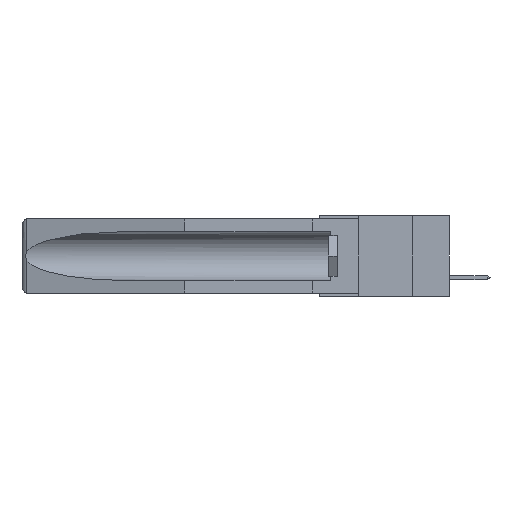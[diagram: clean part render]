
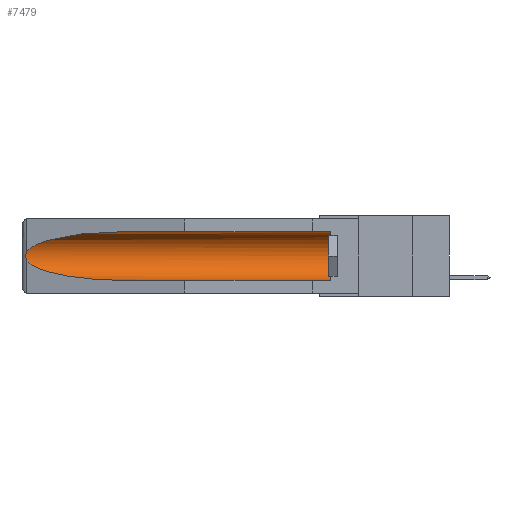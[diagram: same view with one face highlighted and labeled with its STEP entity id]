
A CAD part, left-side view. The second image highlights one B-rep face of the part: STEP entity #7479.
In plain terms, the highlighted cylindrical face has radius 2.857 mm (diameter 5.715 mm), a partial arc.
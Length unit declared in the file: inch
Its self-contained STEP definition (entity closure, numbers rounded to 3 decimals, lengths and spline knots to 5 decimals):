
#168 = CARTESIAN_POINT ( 'NONE',  ( 0.26597, 1.52961, -0.15275 ) ) ;
#580 = LINE ( 'NONE', #3867, #10991 ) ;
#1184 = VERTEX_POINT ( 'NONE', #15081 ) ;
#1246 = FACE_OUTER_BOUND ( 'NONE', #3097, .T. ) ;
#1307 = CARTESIAN_POINT ( 'NONE',  ( 0.26537, 1.52718, -0.19328 ) ) ;
#3097 = EDGE_LOOP ( 'NONE', ( #18067, #24469, #7619, #7277, #23403, #26699 ) ) ;
#3204 = CARTESIAN_POINT ( 'NONE',  ( 0.25451, 1.48313, -0.09465 ) ) ;
#3775 = DIRECTION ( 'NONE',  ( 0., 1., 0. ) ) ;
#3867 = CARTESIAN_POINT ( 'NONE',  ( 0.155, -0.30754, -0.284 ) ) ;
#3916 = CARTESIAN_POINT ( 'NONE',  ( 0.155, 0.126, -0.059 ) ) ;
#4018 = AXIS2_PLACEMENT_3D ( 'NONE', #15516, #21677, #5068 ) ;
#4229 = CARTESIAN_POINT ( 'NONE',  ( 0.155, 0.126, -0.1715 ) ) ;
#4528 = LINE ( 'NONE', #22817, #7834 ) ;
#4541 = CARTESIAN_POINT ( 'NONE',  ( 0.26537, 1.52718, -0.14972 ) ) ;
#4928 = CARTESIAN_POINT ( 'NONE',  ( 0.26537, 1.52718, -0.14972 ) ) ;
#5046 = EDGE_CURVE ( 'NONE', #12075, #1184, #12739, .T. ) ;
#5068 = DIRECTION ( 'NONE',  ( 0., 0., 1. ) ) ;
#5694 = CARTESIAN_POINT ( 'NONE',  ( 0.21114, 1.30732, -0.284 ) ) ;
#5814 = VERTEX_POINT ( 'NONE', #3916 ) ;
#6275 = EDGE_CURVE ( 'NONE', #5814, #20178, #4528, .T. ) ;
#6445 = CARTESIAN_POINT ( 'NONE',  ( 0.2675, 1.53308, -0.16763 ) ) ;
#6728 = CARTESIAN_POINT ( 'NONE',  ( 0.155, 0.126, -0.284 ) ) ;
#6777 = CYLINDRICAL_SURFACE ( 'NONE', #4018, 0.1125 ) ;
#7117 = EDGE_CURVE ( 'NONE', #11679, #12075, #21382, .T. ) ;
#7277 = ORIENTED_EDGE ( 'NONE', *, *, #25145, .F. ) ;
#7479 = ADVANCED_FACE ( 'NONE', ( #1246 ), #6777, .F. ) ;
#7619 = ORIENTED_EDGE ( 'NONE', *, *, #5046, .T. ) ;
#7834 = VECTOR ( 'NONE', #12122, 39.37008 ) ;
#8547 = CARTESIAN_POINT ( 'NONE',  ( 0.26655, 1.53094, -0.18657 ) ) ;
#8723 = CARTESIAN_POINT ( 'NONE',  ( 0.2673, 1.53269, -0.17917 ) ) ;
#9091 = CIRCLE ( 'NONE', #23106, 0.1125 ) ;
#9810 = CARTESIAN_POINT ( 'NONE',  ( 0.26537, 1.52718, -0.19328 ) ) ;
#9898 = CARTESIAN_POINT ( 'NONE',  ( 0.25451, 1.48313, -0.24835 ) ) ;
#10991 = VECTOR ( 'NONE', #3775, 39.37008 ) ;
#11486 = CARTESIAN_POINT ( 'NONE',  ( 0.155, 1.07973, -0.059 ) ) ;
#11679 = VERTEX_POINT ( 'NONE', #19149 ) ;
#12075 = VERTEX_POINT ( 'NONE', #1307 ) ;
#12122 = DIRECTION ( 'NONE',  ( 0., 1., 0. ) ) ;
#12271 = CARTESIAN_POINT ( 'NONE',  ( 0.155, 1.07973, -0.059 ) ) ;
#12561 = CARTESIAN_POINT ( 'NONE',  ( 0.26597, 1.5296, -0.19026 ) ) ;
#12739 =( BOUNDED_CURVE ( )  B_SPLINE_CURVE ( 3, ( #9810, #9898, #5694, #20668 ),
 .UNSPECIFIED., .F., .F. ) 
 B_SPLINE_CURVE_WITH_KNOTS ( ( 4, 4 ),
 ( 0.1948, 1.5708 ),
 .UNSPECIFIED. ) 
 CURVE ( )  GEOMETRIC_REPRESENTATION_ITEM ( )  RATIONAL_B_SPLINE_CURVE ( ( 1., 0.848, 0.848, 1. ) ) 
 REPRESENTATION_ITEM ( '' )  );
#14463 = DIRECTION ( 'NONE',  ( 0., -1., 0. ) ) ;
#14755 = EDGE_CURVE ( 'NONE', #19873, #5814, #9091, .T. ) ;
#15081 = CARTESIAN_POINT ( 'NONE',  ( 0.155, 1.07973, -0.284 ) ) ;
#15288 =( BOUNDED_CURVE ( )  B_SPLINE_CURVE ( 3, ( #11486, #19831, #3204, #4928 ),
 .UNSPECIFIED., .F., .F. ) 
 B_SPLINE_CURVE_WITH_KNOTS ( ( 4, 4 ),
 ( 4.71239, 6.08839 ),
 .UNSPECIFIED. ) 
 CURVE ( )  GEOMETRIC_REPRESENTATION_ITEM ( )  RATIONAL_B_SPLINE_CURVE ( ( 1., 0.848, 0.848, 1. ) ) 
 REPRESENTATION_ITEM ( '' )  );
#15516 = CARTESIAN_POINT ( 'NONE',  ( 0.155, -0.30754, -0.1715 ) ) ;
#18067 = ORIENTED_EDGE ( 'NONE', *, *, #21742, .T. ) ;
#18868 = CARTESIAN_POINT ( 'NONE',  ( 0.26537, 1.52718, -0.19328 ) ) ;
#19046 = CARTESIAN_POINT ( 'NONE',  ( 0.2673, 1.5327, -0.16383 ) ) ;
#19149 = CARTESIAN_POINT ( 'NONE',  ( 0.26537, 1.52718, -0.14972 ) ) ;
#19831 = CARTESIAN_POINT ( 'NONE',  ( 0.21114, 1.30732, -0.059 ) ) ;
#19873 = VERTEX_POINT ( 'NONE', #6728 ) ;
#20178 = VERTEX_POINT ( 'NONE', #12271 ) ;
#20668 = CARTESIAN_POINT ( 'NONE',  ( 0.155, 1.07973, -0.284 ) ) ;
#21015 = DIRECTION ( 'NONE',  ( 0., 0., 1. ) ) ;
#21382 = B_SPLINE_CURVE_WITH_KNOTS ( 'NONE', 3,
 ( #4541, #168, #23331, #19046, #6445, #23244, #8723, #8547, #12561, #18868 ),
 .UNSPECIFIED., .F., .F.,
 ( 4, 2, 2, 2, 4 ),
 ( 0., 0.00029, 0.00058, 0.00087, 0.00117 ),
 .UNSPECIFIED. ) ;
#21677 = DIRECTION ( 'NONE',  ( 0., 1., 0. ) ) ;
#21742 = EDGE_CURVE ( 'NONE', #20178, #11679, #15288, .T. ) ;
#22817 = CARTESIAN_POINT ( 'NONE',  ( 0.155, -0.30754, -0.059 ) ) ;
#23106 = AXIS2_PLACEMENT_3D ( 'NONE', #4229, #14463, #21015 ) ;
#23244 = CARTESIAN_POINT ( 'NONE',  ( 0.2675, 1.53308, -0.17534 ) ) ;
#23331 = CARTESIAN_POINT ( 'NONE',  ( 0.26654, 1.53092, -0.15636 ) ) ;
#23403 = ORIENTED_EDGE ( 'NONE', *, *, #14755, .T. ) ;
#24469 = ORIENTED_EDGE ( 'NONE', *, *, #7117, .T. ) ;
#25145 = EDGE_CURVE ( 'NONE', #19873, #1184, #580, .T. ) ;
#26699 = ORIENTED_EDGE ( 'NONE', *, *, #6275, .T. ) ;
